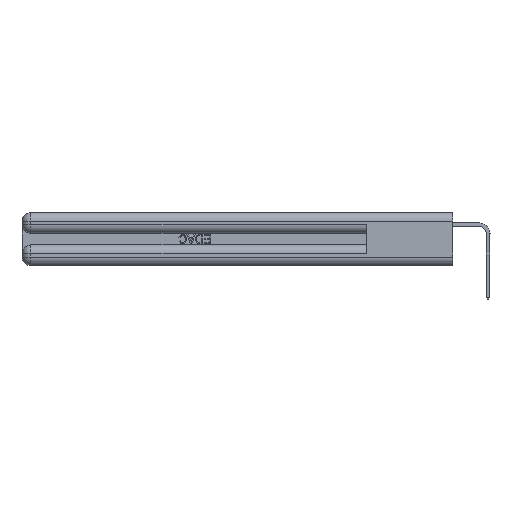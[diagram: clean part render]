
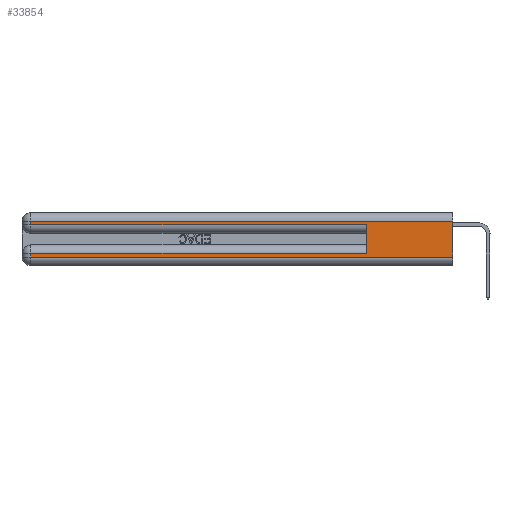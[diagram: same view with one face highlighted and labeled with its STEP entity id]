
A CAD part, left-side view. The second image highlights one B-rep face of the part: STEP entity #33854.
In plain terms, the highlighted planar face has unit normal (-1, 0, 0).
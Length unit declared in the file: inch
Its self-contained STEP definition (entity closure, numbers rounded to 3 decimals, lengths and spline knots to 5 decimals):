
#647 = CARTESIAN_POINT ( 'NONE',  ( 0., 2.94, 0.06 ) ) ;
#1203 = VECTOR ( 'NONE', #46176, 39.37008 ) ;
#1375 = LINE ( 'NONE', #44576, #21953 ) ;
#1840 = CARTESIAN_POINT ( 'NONE',  ( 0., 0., 0.37 ) ) ;
#2063 = DIRECTION ( 'NONE',  ( 0., 1., 0. ) ) ;
#2131 = VECTOR ( 'NONE', #2063, 39.37008 ) ;
#3420 = LINE ( 'NONE', #34818, #2131 ) ;
#4185 = ORIENTED_EDGE ( 'NONE', *, *, #47542, .T. ) ;
#5427 = VERTEX_POINT ( 'NONE', #44395 ) ;
#5435 = ORIENTED_EDGE ( 'NONE', *, *, #9419, .T. ) ;
#6343 = VERTEX_POINT ( 'NONE', #647 ) ;
#6377 = DIRECTION ( 'NONE',  ( 0., 0., -1. ) ) ;
#7185 = VECTOR ( 'NONE', #30003, 39.37008 ) ;
#7709 = VERTEX_POINT ( 'NONE', #50531 ) ;
#9278 = ORIENTED_EDGE ( 'NONE', *, *, #14599, .T. ) ;
#9419 = EDGE_CURVE ( 'NONE', #18451, #51480, #3420, .T. ) ;
#11158 = ORIENTED_EDGE ( 'NONE', *, *, #49461, .F. ) ;
#12013 = CARTESIAN_POINT ( 'NONE',  ( 0., 0., 0.06 ) ) ;
#13622 = CARTESIAN_POINT ( 'NONE',  ( 0., 0.6, 0.145 ) ) ;
#13850 = CARTESIAN_POINT ( 'NONE',  ( 0., 0., 0.37 ) ) ;
#14599 = EDGE_CURVE ( 'NONE', #51480, #41234, #22257, .T. ) ;
#15450 = VERTEX_POINT ( 'NONE', #12013 ) ;
#15940 = VECTOR ( 'NONE', #45161, 39.37008 ) ;
#17632 = VECTOR ( 'NONE', #30352, 39.37008 ) ;
#18015 = PLANE ( 'NONE',  #31569 ) ;
#18451 = VERTEX_POINT ( 'NONE', #50582 ) ;
#19503 = VERTEX_POINT ( 'NONE', #21088 ) ;
#20484 = LINE ( 'NONE', #13622, #1203 ) ;
#20897 = ORIENTED_EDGE ( 'NONE', *, *, #49167, .T. ) ;
#21088 = CARTESIAN_POINT ( 'NONE',  ( 0., 0.6, 0.085 ) ) ;
#21361 = FACE_OUTER_BOUND ( 'NONE', #26794, .T. ) ;
#21622 = CARTESIAN_POINT ( 'NONE',  ( 0., 2.94, 0.285 ) ) ;
#21953 = VECTOR ( 'NONE', #48646, 39.37008 ) ;
#22162 = DIRECTION ( 'NONE',  ( 0., 0., -1. ) ) ;
#22257 = LINE ( 'NONE', #35002, #31824 ) ;
#22374 = VECTOR ( 'NONE', #46745, 39.37008 ) ;
#23634 = LINE ( 'NONE', #1840, #22374 ) ;
#25366 = ORIENTED_EDGE ( 'NONE', *, *, #52158, .T. ) ;
#26794 = EDGE_LOOP ( 'NONE', ( #11158, #5435, #9278, #25366, #27926, #20897, #4185, #31140 ) ) ;
#27747 = LINE ( 'NONE', #38217, #7185 ) ;
#27926 = ORIENTED_EDGE ( 'NONE', *, *, #42814, .F. ) ;
#30003 = DIRECTION ( 'NONE',  ( 0., -1., 0. ) ) ;
#30352 = DIRECTION ( 'NONE',  ( 0., -1., 0. ) ) ;
#31140 = ORIENTED_EDGE ( 'NONE', *, *, #47215, .T. ) ;
#31569 = AXIS2_PLACEMENT_3D ( 'NONE', #13850, #46574, #22162 ) ;
#31824 = VECTOR ( 'NONE', #6377, 39.37008 ) ;
#33854 = ADVANCED_FACE ( 'NONE', ( #21361 ), #18015, .F. ) ;
#34157 = CARTESIAN_POINT ( 'NONE',  ( 0., 2.94, 0.31 ) ) ;
#34818 = CARTESIAN_POINT ( 'NONE',  ( 0., 0., 0.31 ) ) ;
#35002 = CARTESIAN_POINT ( 'NONE',  ( 0., 2.94, 0.37 ) ) ;
#38217 = CARTESIAN_POINT ( 'NONE',  ( 0., 0., 0.06 ) ) ;
#41089 = CARTESIAN_POINT ( 'NONE',  ( 0., 0., 0.085 ) ) ;
#41234 = VERTEX_POINT ( 'NONE', #21622 ) ;
#42814 = EDGE_CURVE ( 'NONE', #19503, #5427, #20484, .T. ) ;
#44395 = CARTESIAN_POINT ( 'NONE',  ( 0., 0.6, 0.285 ) ) ;
#44576 = CARTESIAN_POINT ( 'NONE',  ( 0., 2.94, 0.37 ) ) ;
#45161 = DIRECTION ( 'NONE',  ( 0., 1., 0. ) ) ;
#46176 = DIRECTION ( 'NONE',  ( 0., 0., 1. ) ) ;
#46574 = DIRECTION ( 'NONE',  ( 1., 0., 0. ) ) ;
#46745 = DIRECTION ( 'NONE',  ( 0., 0., -1. ) ) ;
#47215 = EDGE_CURVE ( 'NONE', #6343, #15450, #27747, .T. ) ;
#47542 = EDGE_CURVE ( 'NONE', #7709, #6343, #1375, .T. ) ;
#48531 = LINE ( 'NONE', #41089, #15940 ) ;
#48646 = DIRECTION ( 'NONE',  ( 0., 0., -1. ) ) ;
#49167 = EDGE_CURVE ( 'NONE', #19503, #7709, #48531, .T. ) ;
#49461 = EDGE_CURVE ( 'NONE', #18451, #15450, #23634, .T. ) ;
#50531 = CARTESIAN_POINT ( 'NONE',  ( 0., 2.94, 0.085 ) ) ;
#50582 = CARTESIAN_POINT ( 'NONE',  ( 0., 0., 0.31 ) ) ;
#50803 = CARTESIAN_POINT ( 'NONE',  ( 0., 0., 0.285 ) ) ;
#51414 = LINE ( 'NONE', #50803, #17632 ) ;
#51480 = VERTEX_POINT ( 'NONE', #34157 ) ;
#52158 = EDGE_CURVE ( 'NONE', #41234, #5427, #51414, .T. ) ;
